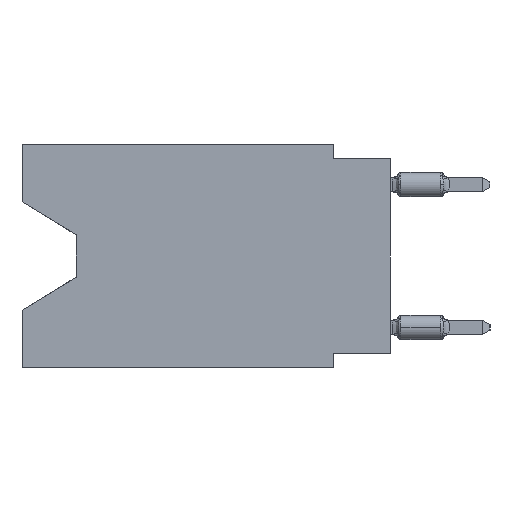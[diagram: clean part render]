
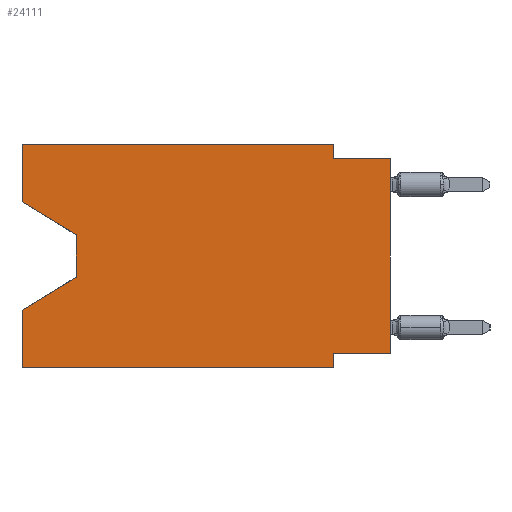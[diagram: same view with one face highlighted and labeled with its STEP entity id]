
A CAD part, left-side view. The second image highlights one B-rep face of the part: STEP entity #24111.
In plain terms, the highlighted planar face has unit normal (-1, 0, 0).
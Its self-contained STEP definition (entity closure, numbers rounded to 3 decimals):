
#131 = CARTESIAN_POINT ( 'NONE',  ( 0., 13.97, -5.893 ) ) ;
#1160 = ORIENTED_EDGE ( 'NONE', *, *, #41718, .T. ) ;
#1404 = DIRECTION ( 'NONE',  ( 0., 0., -1. ) ) ;
#4038 = CARTESIAN_POINT ( 'NONE',  ( 0., 2.54, -9.906 ) ) ;
#6891 = ORIENTED_EDGE ( 'NONE', *, *, #34277, .F. ) ;
#7134 = VERTEX_POINT ( 'NONE', #10657 ) ;
#7335 = VERTEX_POINT ( 'NONE', #12688 ) ;
#7839 = PLANE ( 'NONE',  #22035 ) ;
#8069 = ORIENTED_EDGE ( 'NONE', *, *, #10721, .F. ) ;
#8180 = VECTOR ( 'NONE', #43082, 1000. ) ;
#8388 = VECTOR ( 'NONE', #37416, 1000. ) ;
#8635 = EDGE_LOOP ( 'NONE', ( #41168, #17970, #43586, #6891, #1160, #8069, #11896, #21732, #27981, #17348, #10825, #39492 ) ) ;
#8667 = VERTEX_POINT ( 'NONE', #25617 ) ;
#8916 = VERTEX_POINT ( 'NONE', #4038 ) ;
#9984 = CARTESIAN_POINT ( 'NONE',  ( 0., 16.383, 0. ) ) ;
#10412 = LINE ( 'NONE', #31900, #34547 ) ;
#10579 = VECTOR ( 'NONE', #29492, 1000. ) ;
#10657 = CARTESIAN_POINT ( 'NONE',  ( 0., 16.383, -7.36 ) ) ;
#10721 = EDGE_CURVE ( 'NONE', #8667, #8916, #15198, .T. ) ;
#10825 = ORIENTED_EDGE ( 'NONE', *, *, #27018, .F. ) ;
#11271 = CARTESIAN_POINT ( 'NONE',  ( 0., 16.383, 0. ) ) ;
#11453 = VERTEX_POINT ( 'NONE', #34987 ) ;
#11835 = DIRECTION ( 'NONE',  ( 0., -1., 0. ) ) ;
#11896 = ORIENTED_EDGE ( 'NONE', *, *, #25865, .F. ) ;
#12159 = EDGE_CURVE ( 'NONE', #29780, #20603, #35819, .T. ) ;
#12688 = CARTESIAN_POINT ( 'NONE',  ( 0., 2.54, 0. ) ) ;
#13173 = CARTESIAN_POINT ( 'NONE',  ( 0., 13.97, -4.013 ) ) ;
#14327 = CARTESIAN_POINT ( 'NONE',  ( 0., 16.383, 0. ) ) ;
#14559 = CARTESIAN_POINT ( 'NONE',  ( 0., 2.54, -0.635 ) ) ;
#14841 = CARTESIAN_POINT ( 'NONE',  ( 0., 16.383, 0. ) ) ;
#15066 = VECTOR ( 'NONE', #11835, 1000. ) ;
#15198 = LINE ( 'NONE', #28670, #8180 ) ;
#15991 = LINE ( 'NONE', #16449, #20901 ) ;
#16449 = CARTESIAN_POINT ( 'NONE',  ( 0., 16.383, -2.546 ) ) ;
#16618 = DIRECTION ( 'NONE',  ( 0., 0., 1. ) ) ;
#17142 = EDGE_CURVE ( 'NONE', #27069, #7134, #31459, .T. ) ;
#17348 = ORIENTED_EDGE ( 'NONE', *, *, #39383, .F. ) ;
#17970 = ORIENTED_EDGE ( 'NONE', *, *, #40819, .T. ) ;
#18259 = DIRECTION ( 'NONE',  ( 0., 0., 1. ) ) ;
#18458 = CARTESIAN_POINT ( 'NONE',  ( 0., 0., -0.635 ) ) ;
#18921 = CARTESIAN_POINT ( 'NONE',  ( 0., 16.383, -9.906 ) ) ;
#19592 = LINE ( 'NONE', #36739, #37382 ) ;
#20603 = VERTEX_POINT ( 'NONE', #30123 ) ;
#20901 = VECTOR ( 'NONE', #26505, 1000. ) ;
#21732 = ORIENTED_EDGE ( 'NONE', *, *, #25806, .T. ) ;
#22035 = AXIS2_PLACEMENT_3D ( 'NONE', #11271, #39840, #1404 ) ;
#23316 = LINE ( 'NONE', #30166, #10579 ) ;
#23918 = DIRECTION ( 'NONE',  ( 0., 1., 0. ) ) ;
#24111 = ADVANCED_FACE ( 'NONE', ( #39586 ), #7839, .F. ) ;
#24240 = CARTESIAN_POINT ( 'NONE',  ( 0., 0., -9.271 ) ) ;
#25413 = CARTESIAN_POINT ( 'NONE',  ( 0., 16.383, -2.546 ) ) ;
#25617 = CARTESIAN_POINT ( 'NONE',  ( 0., 2.54, -9.271 ) ) ;
#25766 = DIRECTION ( 'NONE',  ( 0., 0., -1. ) ) ;
#25806 = EDGE_CURVE ( 'NONE', #38889, #20603, #19592, .T. ) ;
#25865 = EDGE_CURVE ( 'NONE', #38889, #8667, #10412, .T. ) ;
#26049 = LINE ( 'NONE', #14841, #31679 ) ;
#26505 = DIRECTION ( 'NONE',  ( 0., -0.855, -0.519 ) ) ;
#26690 = VECTOR ( 'NONE', #30987, 1000. ) ;
#27018 = EDGE_CURVE ( 'NONE', #39525, #7335, #27351, .T. ) ;
#27069 = VERTEX_POINT ( 'NONE', #34427 ) ;
#27351 = LINE ( 'NONE', #9984, #8388 ) ;
#27981 = ORIENTED_EDGE ( 'NONE', *, *, #12159, .F. ) ;
#28670 = CARTESIAN_POINT ( 'NONE',  ( 0., 2.54, -9.906 ) ) ;
#28977 = DIRECTION ( 'NONE',  ( 0., -1., 0. ) ) ;
#29492 = DIRECTION ( 'NONE',  ( 0., 0., 1. ) ) ;
#29780 = VERTEX_POINT ( 'NONE', #14559 ) ;
#30123 = CARTESIAN_POINT ( 'NONE',  ( 0., 0., -0.635 ) ) ;
#30166 = CARTESIAN_POINT ( 'NONE',  ( 0., 16.383, 0. ) ) ;
#30666 = VERTEX_POINT ( 'NONE', #35471 ) ;
#30749 = LINE ( 'NONE', #13173, #26690 ) ;
#30987 = DIRECTION ( 'NONE',  ( 0., 0., -1. ) ) ;
#31187 = EDGE_CURVE ( 'NONE', #31777, #39525, #26049, .T. ) ;
#31459 = LINE ( 'NONE', #131, #32867 ) ;
#31679 = VECTOR ( 'NONE', #18259, 1000. ) ;
#31777 = VERTEX_POINT ( 'NONE', #25413 ) ;
#31900 = CARTESIAN_POINT ( 'NONE',  ( 0., 0., -9.271 ) ) ;
#32867 = VECTOR ( 'NONE', #38573, 1000. ) ;
#34277 = EDGE_CURVE ( 'NONE', #30666, #7134, #23316, .T. ) ;
#34427 = CARTESIAN_POINT ( 'NONE',  ( 0., 13.97, -5.893 ) ) ;
#34547 = VECTOR ( 'NONE', #23918, 1000. ) ;
#34987 = CARTESIAN_POINT ( 'NONE',  ( 0., 13.97, -4.013 ) ) ;
#35471 = CARTESIAN_POINT ( 'NONE',  ( 0., 16.383, -9.906 ) ) ;
#35614 = CARTESIAN_POINT ( 'NONE',  ( 0., 2.54, 0. ) ) ;
#35819 = LINE ( 'NONE', #18458, #38173 ) ;
#35820 = LINE ( 'NONE', #18921, #15066 ) ;
#36070 = LINE ( 'NONE', #35614, #43465 ) ;
#36739 = CARTESIAN_POINT ( 'NONE',  ( 0., 0., 0. ) ) ;
#37382 = VECTOR ( 'NONE', #16618, 1000. ) ;
#37416 = DIRECTION ( 'NONE',  ( 0., -1., 0. ) ) ;
#38173 = VECTOR ( 'NONE', #28977, 1000. ) ;
#38573 = DIRECTION ( 'NONE',  ( 0., 0.855, -0.519 ) ) ;
#38889 = VERTEX_POINT ( 'NONE', #24240 ) ;
#39383 = EDGE_CURVE ( 'NONE', #7335, #29780, #36070, .T. ) ;
#39492 = ORIENTED_EDGE ( 'NONE', *, *, #31187, .F. ) ;
#39525 = VERTEX_POINT ( 'NONE', #14327 ) ;
#39586 = FACE_OUTER_BOUND ( 'NONE', #8635, .T. ) ;
#39840 = DIRECTION ( 'NONE',  ( 1., 0., 0. ) ) ;
#40819 = EDGE_CURVE ( 'NONE', #11453, #27069, #30749, .T. ) ;
#41168 = ORIENTED_EDGE ( 'NONE', *, *, #41512, .T. ) ;
#41512 = EDGE_CURVE ( 'NONE', #31777, #11453, #15991, .T. ) ;
#41718 = EDGE_CURVE ( 'NONE', #30666, #8916, #35820, .T. ) ;
#43082 = DIRECTION ( 'NONE',  ( 0., 0., -1. ) ) ;
#43465 = VECTOR ( 'NONE', #25766, 1000. ) ;
#43586 = ORIENTED_EDGE ( 'NONE', *, *, #17142, .T. ) ;
